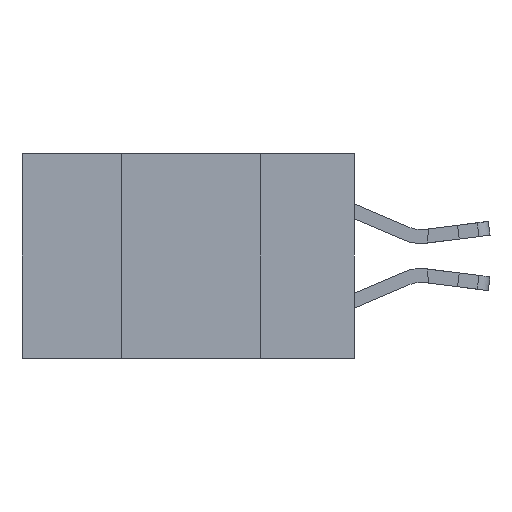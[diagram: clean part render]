
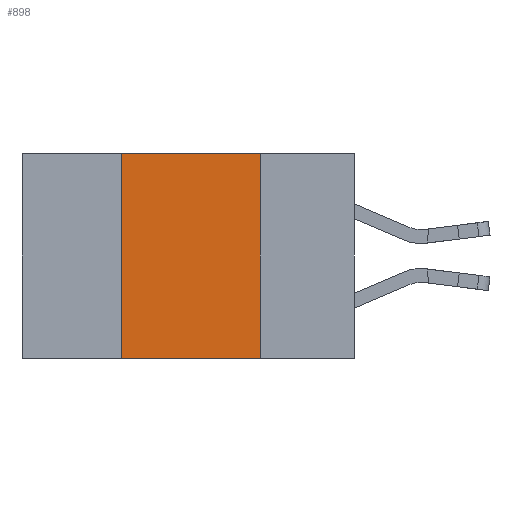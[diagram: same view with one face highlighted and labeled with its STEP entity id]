
A CAD part, left-side view. The second image highlights one B-rep face of the part: STEP entity #898.
In plain terms, the highlighted planar face has unit normal (-1, 0, 0).
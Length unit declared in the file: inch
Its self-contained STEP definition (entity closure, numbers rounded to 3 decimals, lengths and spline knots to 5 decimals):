
#25 = LINE ( 'NONE', #9456, #14536 ) ;
#41 = VERTEX_POINT ( 'NONE', #3267 ) ;
#146 = AXIS2_PLACEMENT_3D ( 'NONE', #6547, #17188, #9194 ) ;
#472 = ORIENTED_EDGE ( 'NONE', *, *, #3697, .F. ) ;
#533 = EDGE_CURVE ( 'NONE', #41, #7933, #15158, .T. ) ;
#898 = ADVANCED_FACE ( 'NONE', ( #12794 ), #16043, .F. ) ;
#907 = CARTESIAN_POINT ( 'NONE',  ( 0., 0.42, 0. ) ) ;
#1370 = LINE ( 'NONE', #17698, #4827 ) ;
#1466 = CARTESIAN_POINT ( 'NONE',  ( 0., 0.42, 0. ) ) ;
#1596 = VECTOR ( 'NONE', #9952, 39.37008 ) ;
#1980 = CARTESIAN_POINT ( 'NONE',  ( 0., 0.17, -0.37 ) ) ;
#2406 = EDGE_LOOP ( 'NONE', ( #4686, #472, #13883, #16445 ) ) ;
#2569 = CARTESIAN_POINT ( 'NONE',  ( 0., 0.17, 0. ) ) ;
#2838 = DIRECTION ( 'NONE',  ( 0., -1., 0. ) ) ;
#2914 = CARTESIAN_POINT ( 'NONE',  ( 0., 0.6, -0.37 ) ) ;
#3267 = CARTESIAN_POINT ( 'NONE',  ( 0., 0.42, -0.37 ) ) ;
#3697 = EDGE_CURVE ( 'NONE', #12186, #13957, #1370, .T. ) ;
#4686 = ORIENTED_EDGE ( 'NONE', *, *, #8831, .F. ) ;
#4827 = VECTOR ( 'NONE', #16255, 39.37008 ) ;
#6547 = CARTESIAN_POINT ( 'NONE',  ( 0., 0.6, 0. ) ) ;
#7933 = VERTEX_POINT ( 'NONE', #1980 ) ;
#8831 = EDGE_CURVE ( 'NONE', #13957, #7933, #25, .T. ) ;
#9194 = DIRECTION ( 'NONE',  ( 0., 0., -1. ) ) ;
#9456 = CARTESIAN_POINT ( 'NONE',  ( 0., 0.17, 0. ) ) ;
#9952 = DIRECTION ( 'NONE',  ( 0., 0., 1. ) ) ;
#11522 = VECTOR ( 'NONE', #2838, 39.37008 ) ;
#12186 = VERTEX_POINT ( 'NONE', #907 ) ;
#12794 = FACE_OUTER_BOUND ( 'NONE', #2406, .T. ) ;
#13883 = ORIENTED_EDGE ( 'NONE', *, *, #17152, .F. ) ;
#13957 = VERTEX_POINT ( 'NONE', #2569 ) ;
#14536 = VECTOR ( 'NONE', #17650, 39.37008 ) ;
#15158 = LINE ( 'NONE', #2914, #11522 ) ;
#16020 = LINE ( 'NONE', #1466, #1596 ) ;
#16043 = PLANE ( 'NONE',  #146 ) ;
#16255 = DIRECTION ( 'NONE',  ( 0., -1., 0. ) ) ;
#16445 = ORIENTED_EDGE ( 'NONE', *, *, #533, .T. ) ;
#17152 = EDGE_CURVE ( 'NONE', #41, #12186, #16020, .T. ) ;
#17188 = DIRECTION ( 'NONE',  ( 1., 0., 0. ) ) ;
#17650 = DIRECTION ( 'NONE',  ( 0., 0., -1. ) ) ;
#17698 = CARTESIAN_POINT ( 'NONE',  ( 0., 0.6, 0. ) ) ;
